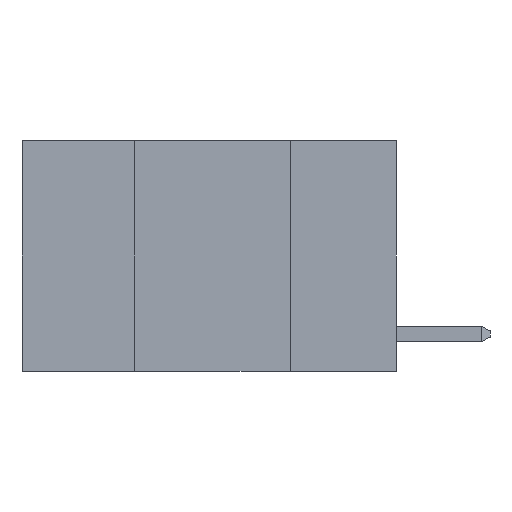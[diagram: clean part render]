
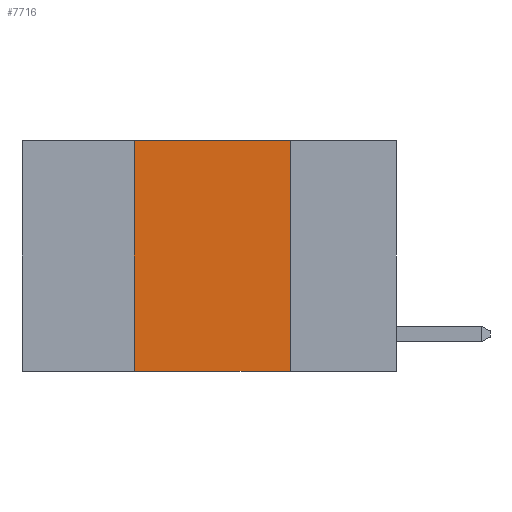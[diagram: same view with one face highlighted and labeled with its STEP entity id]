
A CAD part, left-side view. The second image highlights one B-rep face of the part: STEP entity #7716.
In plain terms, the highlighted planar face has unit normal (-1, 0, 0).
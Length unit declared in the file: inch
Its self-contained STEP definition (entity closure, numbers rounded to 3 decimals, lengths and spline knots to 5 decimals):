
#111 = VERTEX_POINT ( 'NONE', #383 ) ;
#336 = LINE ( 'NONE', #6519, #2334 ) ;
#383 = CARTESIAN_POINT ( 'NONE',  ( 0., 0.17, 0. ) ) ;
#679 = CARTESIAN_POINT ( 'NONE',  ( 0., 0.17, 0. ) ) ;
#1224 = EDGE_CURVE ( 'NONE', #6718, #111, #4036, .T. ) ;
#1737 = CARTESIAN_POINT ( 'NONE',  ( 0., 0.42, 0. ) ) ;
#1968 = DIRECTION ( 'NONE',  ( 0., -1., 0. ) ) ;
#2001 = VECTOR ( 'NONE', #1968, 39.37008 ) ;
#2073 = VERTEX_POINT ( 'NONE', #8286 ) ;
#2334 = VECTOR ( 'NONE', #3422, 39.37008 ) ;
#2352 = EDGE_CURVE ( 'NONE', #5765, #2073, #336, .T. ) ;
#2373 = ORIENTED_EDGE ( 'NONE', *, *, #2352, .T. ) ;
#2647 = CARTESIAN_POINT ( 'NONE',  ( 0., 0.42, 0. ) ) ;
#2847 = EDGE_CURVE ( 'NONE', #5765, #6718, #9568, .T. ) ;
#3350 = LINE ( 'NONE', #679, #5140 ) ;
#3422 = DIRECTION ( 'NONE',  ( 0., -1., 0. ) ) ;
#3779 = ORIENTED_EDGE ( 'NONE', *, *, #1224, .F. ) ;
#3862 = DIRECTION ( 'NONE',  ( 1., 0., 0. ) ) ;
#4036 = LINE ( 'NONE', #4997, #2001 ) ;
#4327 = FACE_OUTER_BOUND ( 'NONE', #6499, .T. ) ;
#4939 = DIRECTION ( 'NONE',  ( 0., 0., 1. ) ) ;
#4997 = CARTESIAN_POINT ( 'NONE',  ( 0., 0.6, 0. ) ) ;
#5140 = VECTOR ( 'NONE', #6753, 39.37008 ) ;
#5765 = VERTEX_POINT ( 'NONE', #8924 ) ;
#5775 = EDGE_CURVE ( 'NONE', #111, #2073, #3350, .T. ) ;
#6499 = EDGE_LOOP ( 'NONE', ( #8577, #3779, #8133, #2373 ) ) ;
#6519 = CARTESIAN_POINT ( 'NONE',  ( 0., 0.6, -0.37 ) ) ;
#6718 = VERTEX_POINT ( 'NONE', #1737 ) ;
#6753 = DIRECTION ( 'NONE',  ( 0., 0., -1. ) ) ;
#6852 = CARTESIAN_POINT ( 'NONE',  ( 0., 0.6, 0. ) ) ;
#7627 = VECTOR ( 'NONE', #4939, 39.37008 ) ;
#7716 = ADVANCED_FACE ( 'NONE', ( #4327 ), #8323, .F. ) ;
#8133 = ORIENTED_EDGE ( 'NONE', *, *, #2847, .F. ) ;
#8286 = CARTESIAN_POINT ( 'NONE',  ( 0., 0.17, -0.37 ) ) ;
#8323 = PLANE ( 'NONE',  #9702 ) ;
#8577 = ORIENTED_EDGE ( 'NONE', *, *, #5775, .F. ) ;
#8924 = CARTESIAN_POINT ( 'NONE',  ( 0., 0.42, -0.37 ) ) ;
#9048 = DIRECTION ( 'NONE',  ( 0., 0., -1. ) ) ;
#9568 = LINE ( 'NONE', #2647, #7627 ) ;
#9702 = AXIS2_PLACEMENT_3D ( 'NONE', #6852, #3862, #9048 ) ;
